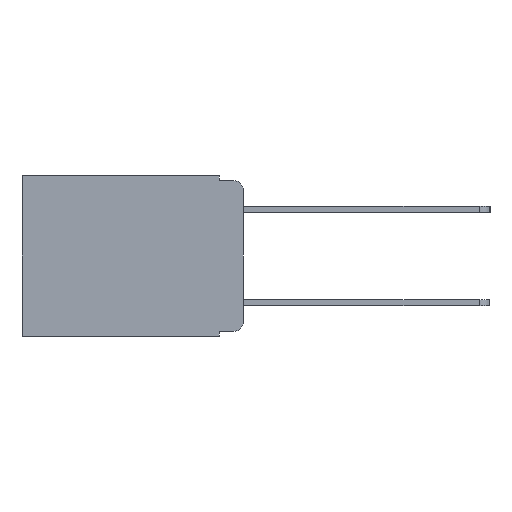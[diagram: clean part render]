
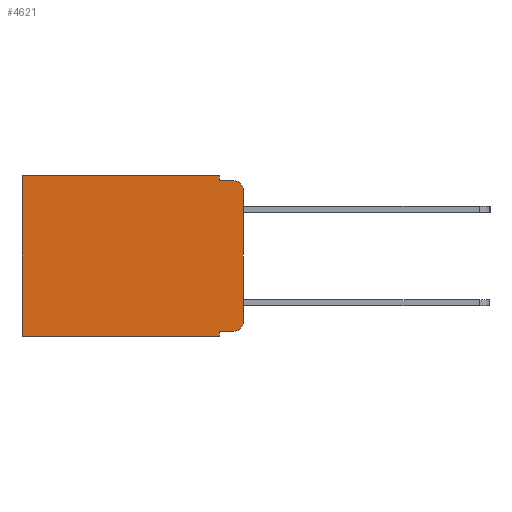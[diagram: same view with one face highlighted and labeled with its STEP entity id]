
A CAD part, left-side view. The second image highlights one B-rep face of the part: STEP entity #4621.
In plain terms, the highlighted planar face has unit normal (-1, 0, 0).
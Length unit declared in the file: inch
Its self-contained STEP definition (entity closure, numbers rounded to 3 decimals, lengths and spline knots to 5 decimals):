
#96 = ORIENTED_EDGE ( 'NONE', *, *, #8977, .T. ) ;
#110 = DIRECTION ( 'NONE',  ( 0., -1., 0. ) ) ;
#211 = VERTEX_POINT ( 'NONE', #11424 ) ;
#447 = ORIENTED_EDGE ( 'NONE', *, *, #5716, .F. ) ;
#471 = VECTOR ( 'NONE', #110, 39.37008 ) ;
#591 = CARTESIAN_POINT ( 'NONE',  ( 0.298, 0.473, 0. ) ) ;
#721 = CARTESIAN_POINT ( 'NONE',  ( 0.298, 0., -0.03 ) ) ;
#841 = CARTESIAN_POINT ( 'NONE',  ( 0.298, 0., -0.343 ) ) ;
#951 = VECTOR ( 'NONE', #8928, 39.37008 ) ;
#1410 = VECTOR ( 'NONE', #10981, 39.37008 ) ;
#1445 = EDGE_CURVE ( 'NONE', #211, #2710, #8995, .T. ) ;
#1577 = DIRECTION ( 'NONE',  ( 0., 0., -1. ) ) ;
#1749 = CARTESIAN_POINT ( 'NONE',  ( 0.298, 0.051, -0.01 ) ) ;
#1823 = EDGE_CURVE ( 'NONE', #7365, #9642, #7419, .T. ) ;
#1854 = CARTESIAN_POINT ( 'NONE',  ( 0.298, 0.02, -0.333 ) ) ;
#2135 = VERTEX_POINT ( 'NONE', #4295 ) ;
#2237 = EDGE_LOOP ( 'NONE', ( #7475, #7214, #7593, #447, #96, #5328, #5039, #7353, #11017, #7107 ) ) ;
#2338 = CIRCLE ( 'NONE', #5654, 0.02 ) ;
#2347 = EDGE_CURVE ( 'NONE', #5156, #9642, #9088, .T. ) ;
#2592 = VERTEX_POINT ( 'NONE', #10923 ) ;
#2710 = VERTEX_POINT ( 'NONE', #7765 ) ;
#2964 = DIRECTION ( 'NONE',  ( 0., 0., -1. ) ) ;
#3058 = VECTOR ( 'NONE', #3192, 39.37008 ) ;
#3106 = CARTESIAN_POINT ( 'NONE',  ( 0.298, 0., 0. ) ) ;
#3192 = DIRECTION ( 'NONE',  ( 0., 0., -1. ) ) ;
#3583 = LINE ( 'NONE', #10601, #7702 ) ;
#3604 = LINE ( 'NONE', #591, #951 ) ;
#3713 = CARTESIAN_POINT ( 'NONE',  ( 0.298, 0.02, -0.03 ) ) ;
#3854 = EDGE_CURVE ( 'NONE', #2135, #2710, #3604, .T. ) ;
#3873 = VERTEX_POINT ( 'NONE', #1749 ) ;
#3918 = CARTESIAN_POINT ( 'NONE',  ( 0.298, 0.051, -0.333 ) ) ;
#4295 = CARTESIAN_POINT ( 'NONE',  ( 0.298, 0.473, 0. ) ) ;
#4534 = LINE ( 'NONE', #3106, #6650 ) ;
#4580 = VECTOR ( 'NONE', #4820, 39.37008 ) ;
#4621 = ADVANCED_FACE ( 'NONE', ( #8661 ), #7418, .F. ) ;
#4643 = DIRECTION ( 'NONE',  ( 0., 0., -1. ) ) ;
#4700 = EDGE_CURVE ( 'NONE', #9538, #211, #3583, .T. ) ;
#4820 = DIRECTION ( 'NONE',  ( 0., -1., 0. ) ) ;
#4931 = DIRECTION ( 'NONE',  ( 0., 0., -1. ) ) ;
#5039 = ORIENTED_EDGE ( 'NONE', *, *, #1445, .F. ) ;
#5156 = VERTEX_POINT ( 'NONE', #721 ) ;
#5328 = ORIENTED_EDGE ( 'NONE', *, *, #3854, .T. ) ;
#5330 = EDGE_CURVE ( 'NONE', #9538, #7365, #11140, .T. ) ;
#5654 = AXIS2_PLACEMENT_3D ( 'NONE', #3713, #9587, #4643 ) ;
#5712 = CARTESIAN_POINT ( 'NONE',  ( 0.298, 0., 0. ) ) ;
#5716 = EDGE_CURVE ( 'NONE', #7622, #3873, #8644, .T. ) ;
#5935 = CARTESIAN_POINT ( 'NONE',  ( 0.298, 0.051, -0.01 ) ) ;
#5965 = CARTESIAN_POINT ( 'NONE',  ( 0.298, 0., 0. ) ) ;
#6222 = CARTESIAN_POINT ( 'NONE',  ( 0.298, 0.051, 0. ) ) ;
#6650 = VECTOR ( 'NONE', #9065, 39.37008 ) ;
#6744 = DIRECTION ( 'NONE',  ( -1., 0., 0. ) ) ;
#7107 = ORIENTED_EDGE ( 'NONE', *, *, #1823, .T. ) ;
#7214 = ORIENTED_EDGE ( 'NONE', *, *, #9477, .T. ) ;
#7304 = DIRECTION ( 'NONE',  ( 0., 1., 0. ) ) ;
#7353 = ORIENTED_EDGE ( 'NONE', *, *, #4700, .F. ) ;
#7365 = VERTEX_POINT ( 'NONE', #1854 ) ;
#7418 = PLANE ( 'NONE',  #7968 ) ;
#7419 = CIRCLE ( 'NONE', #10352, 0.02 ) ;
#7431 = VECTOR ( 'NONE', #7304, 39.37008 ) ;
#7475 = ORIENTED_EDGE ( 'NONE', *, *, #2347, .F. ) ;
#7593 = ORIENTED_EDGE ( 'NONE', *, *, #11276, .F. ) ;
#7622 = VERTEX_POINT ( 'NONE', #7726 ) ;
#7702 = VECTOR ( 'NONE', #4931, 39.37008 ) ;
#7726 = CARTESIAN_POINT ( 'NONE',  ( 0.298, 0.051, 0. ) ) ;
#7765 = CARTESIAN_POINT ( 'NONE',  ( 0.298, 0.473, -0.343 ) ) ;
#7968 = AXIS2_PLACEMENT_3D ( 'NONE', #5712, #8166, #2964 ) ;
#8166 = DIRECTION ( 'NONE',  ( 1., 0., 0. ) ) ;
#8425 = CARTESIAN_POINT ( 'NONE',  ( 0.298, 0.02, -0.313 ) ) ;
#8644 = LINE ( 'NONE', #6222, #1410 ) ;
#8661 = FACE_OUTER_BOUND ( 'NONE', #2237, .T. ) ;
#8928 = DIRECTION ( 'NONE',  ( 0., 0., -1. ) ) ;
#8957 = CARTESIAN_POINT ( 'NONE',  ( 0.298, 0., -0.313 ) ) ;
#8977 = EDGE_CURVE ( 'NONE', #7622, #2135, #4534, .T. ) ;
#8995 = LINE ( 'NONE', #841, #7431 ) ;
#9065 = DIRECTION ( 'NONE',  ( 0., 1., 0. ) ) ;
#9088 = LINE ( 'NONE', #5965, #3058 ) ;
#9477 = EDGE_CURVE ( 'NONE', #5156, #2592, #2338, .T. ) ;
#9538 = VERTEX_POINT ( 'NONE', #11244 ) ;
#9587 = DIRECTION ( 'NONE',  ( -1., 0., 0. ) ) ;
#9642 = VERTEX_POINT ( 'NONE', #8957 ) ;
#9888 = LINE ( 'NONE', #5935, #471 ) ;
#10352 = AXIS2_PLACEMENT_3D ( 'NONE', #8425, #6744, #1577 ) ;
#10601 = CARTESIAN_POINT ( 'NONE',  ( 0.298, 0.051, 0. ) ) ;
#10923 = CARTESIAN_POINT ( 'NONE',  ( 0.298, 0.02, -0.01 ) ) ;
#10981 = DIRECTION ( 'NONE',  ( 0., 0., -1. ) ) ;
#11017 = ORIENTED_EDGE ( 'NONE', *, *, #5330, .T. ) ;
#11140 = LINE ( 'NONE', #3918, #4580 ) ;
#11244 = CARTESIAN_POINT ( 'NONE',  ( 0.298, 0.051, -0.333 ) ) ;
#11276 = EDGE_CURVE ( 'NONE', #3873, #2592, #9888, .T. ) ;
#11424 = CARTESIAN_POINT ( 'NONE',  ( 0.298, 0.051, -0.343 ) ) ;
